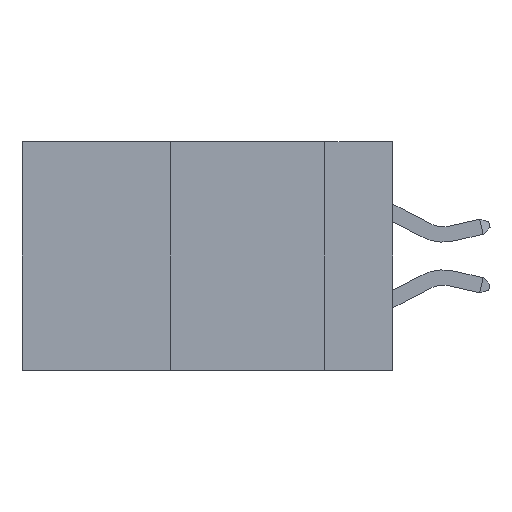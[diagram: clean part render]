
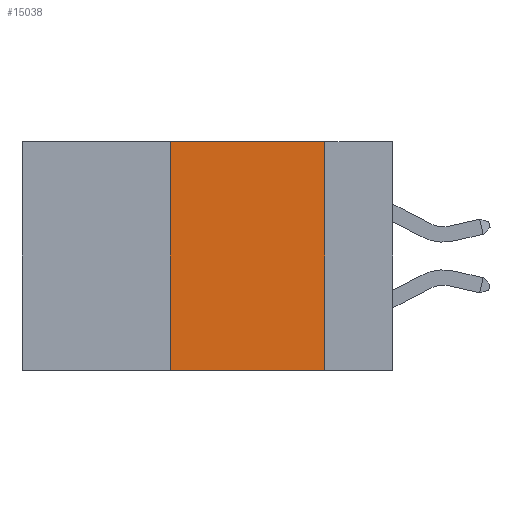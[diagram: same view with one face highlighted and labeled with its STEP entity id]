
A CAD part, left-side view. The second image highlights one B-rep face of the part: STEP entity #15038.
In plain terms, the highlighted planar face has unit normal (-1, 0, 0).
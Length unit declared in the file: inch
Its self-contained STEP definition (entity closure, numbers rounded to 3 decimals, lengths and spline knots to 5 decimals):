
#447 = LINE ( 'NONE', #5387, #6701 ) ;
#991 = FACE_OUTER_BOUND ( 'NONE', #1305, .T. ) ;
#1305 = EDGE_LOOP ( 'NONE', ( #11591, #5113, #13036, #8978 ) ) ;
#1385 = DIRECTION ( 'NONE',  ( 1., 0., 0. ) ) ;
#1408 = EDGE_CURVE ( 'NONE', #8229, #6739, #12901, .T. ) ;
#1661 = EDGE_CURVE ( 'NONE', #6739, #10296, #7782, .T. ) ;
#2693 = DIRECTION ( 'NONE',  ( 0., -1., 0. ) ) ;
#2766 = EDGE_CURVE ( 'NONE', #4643, #10296, #12656, .T. ) ;
#2837 = VECTOR ( 'NONE', #14894, 39.37008 ) ;
#4265 = CARTESIAN_POINT ( 'NONE',  ( 0., 0.11, -0.37 ) ) ;
#4366 = EDGE_CURVE ( 'NONE', #4643, #8229, #447, .T. ) ;
#4643 = VERTEX_POINT ( 'NONE', #9482 ) ;
#5113 = ORIENTED_EDGE ( 'NONE', *, *, #1408, .F. ) ;
#5212 = CARTESIAN_POINT ( 'NONE',  ( 0., 0.6, 0. ) ) ;
#5307 = VECTOR ( 'NONE', #6502, 39.37008 ) ;
#5387 = CARTESIAN_POINT ( 'NONE',  ( 0., 0.36, 0. ) ) ;
#5528 = CARTESIAN_POINT ( 'NONE',  ( 0., 0.36, 0. ) ) ;
#6502 = DIRECTION ( 'NONE',  ( 0., -1., 0. ) ) ;
#6701 = VECTOR ( 'NONE', #10053, 39.37008 ) ;
#6739 = VERTEX_POINT ( 'NONE', #11644 ) ;
#7409 = CARTESIAN_POINT ( 'NONE',  ( 0., 0.6, 0. ) ) ;
#7782 = LINE ( 'NONE', #9963, #2837 ) ;
#8229 = VERTEX_POINT ( 'NONE', #5528 ) ;
#8978 = ORIENTED_EDGE ( 'NONE', *, *, #2766, .T. ) ;
#9482 = CARTESIAN_POINT ( 'NONE',  ( 0., 0.36, -0.37 ) ) ;
#9869 = DIRECTION ( 'NONE',  ( 0., 0., -1. ) ) ;
#9963 = CARTESIAN_POINT ( 'NONE',  ( 0., 0.11, 0. ) ) ;
#10053 = DIRECTION ( 'NONE',  ( 0., 0., 1. ) ) ;
#10296 = VERTEX_POINT ( 'NONE', #4265 ) ;
#11500 = VECTOR ( 'NONE', #2693, 39.37008 ) ;
#11591 = ORIENTED_EDGE ( 'NONE', *, *, #1661, .F. ) ;
#11644 = CARTESIAN_POINT ( 'NONE',  ( 0., 0.11, 0. ) ) ;
#12142 = PLANE ( 'NONE',  #13357 ) ;
#12656 = LINE ( 'NONE', #13175, #11500 ) ;
#12901 = LINE ( 'NONE', #5212, #5307 ) ;
#13036 = ORIENTED_EDGE ( 'NONE', *, *, #4366, .F. ) ;
#13175 = CARTESIAN_POINT ( 'NONE',  ( 0., 0.6, -0.37 ) ) ;
#13357 = AXIS2_PLACEMENT_3D ( 'NONE', #7409, #1385, #9869 ) ;
#14894 = DIRECTION ( 'NONE',  ( 0., 0., -1. ) ) ;
#15038 = ADVANCED_FACE ( 'NONE', ( #991 ), #12142, .F. ) ;
